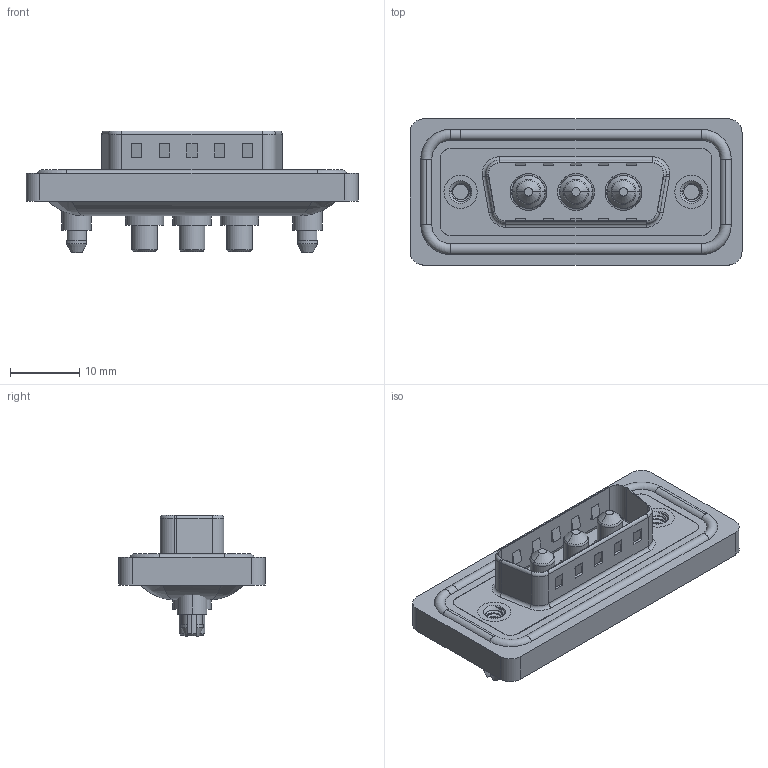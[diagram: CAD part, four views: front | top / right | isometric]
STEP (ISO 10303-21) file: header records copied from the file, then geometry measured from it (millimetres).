
FILE_DESCRIPTION (( 'STEP AP203' ), '1' );
FILE_NAME ('627W3W3-324-4N5.STEP', '2024-03-19T17:54:51', ( '' ), ( '' ), 'SwSTEP 2.0', 'SolidWorks 2023', '' );
FILE_SCHEMA (( 'CONFIG_CONTROL_DESIGN' ));
Length unit declared in the file: millimetre
Products named in the file (7): 627Combo Housing_3W3; 627W3W3-324-4N5; 627Combo Shell Front_15 Contacts; Power Pin_40A S; 627Combo Shell Rear_15 Contacts; 627Combo Waterproof Housing_15 Contacts; 627Combo Threaded Boardlock_5
Assembly tree (9 placements, depth 2):
  627W3W3-324-4N5
    627Combo Housing_3W3
    627Combo Waterproof Housing_15 Contacts
    627Combo Shell Rear_15 Contacts
    627Combo Shell Front_15 Contacts
    627Combo Threaded Boardlock_5  x2
    Power Pin_40A S  x3
Bounding box: 47.9 x 21.1 x 17.6 mm (x, y, z)
Volume: 5774.7 mm3; surface area: 9119.2 mm2
Topology: 13 solids, 13 shells, 614 faces, 1507 edges, 945 vertices
Faces by surface type: cylinder 273, plane 223, torus 70, cone 35, bspline 13
Entity records: 17297 total; most frequent: CARTESIAN_POINT 4636, DIRECTION 2567, ORIENTED_EDGE 2424, EDGE_CURVE 1212, AXIS2_PLACEMENT_3D 959, VERTEX_POINT 766, VECTOR 649, LINE 649
